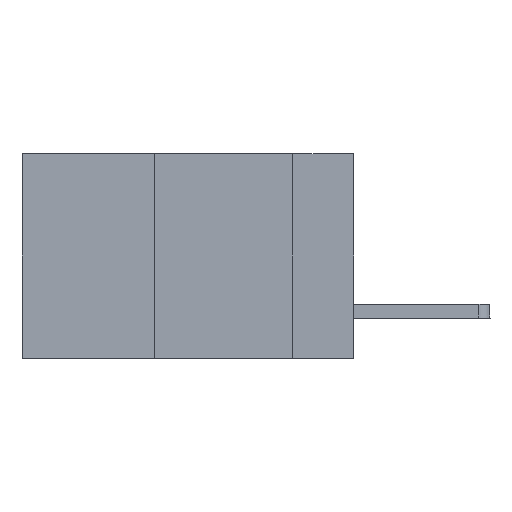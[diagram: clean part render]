
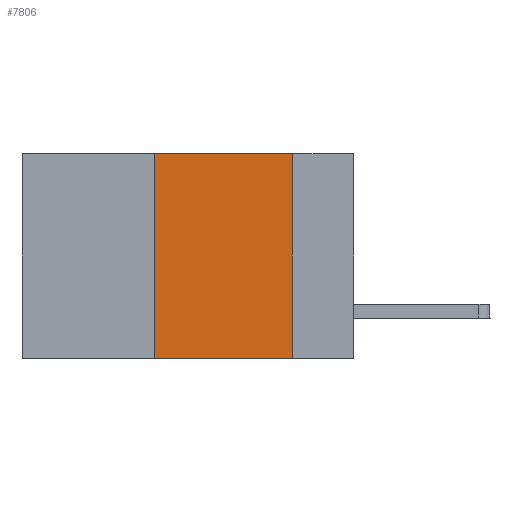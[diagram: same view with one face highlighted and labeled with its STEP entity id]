
A CAD part, left-side view. The second image highlights one B-rep face of the part: STEP entity #7806.
In plain terms, the highlighted planar face has unit normal (-1, 0, 0).
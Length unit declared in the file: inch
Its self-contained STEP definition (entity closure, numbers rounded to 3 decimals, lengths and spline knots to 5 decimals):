
#209 = CARTESIAN_POINT ( 'NONE',  ( 0., 0.11, 0. ) ) ;
#317 = CARTESIAN_POINT ( 'NONE',  ( 0., 0.6, -0.37 ) ) ;
#712 = VECTOR ( 'NONE', #8814, 39.37008 ) ;
#932 = FACE_OUTER_BOUND ( 'NONE', #9823, .T. ) ;
#1489 = LINE ( 'NONE', #3153, #5176 ) ;
#2390 = DIRECTION ( 'NONE',  ( 0., -1., 0. ) ) ;
#2405 = ORIENTED_EDGE ( 'NONE', *, *, #6902, .T. ) ;
#2842 = VERTEX_POINT ( 'NONE', #6450 ) ;
#3153 = CARTESIAN_POINT ( 'NONE',  ( 0., 0.36, 0. ) ) ;
#3265 = CARTESIAN_POINT ( 'NONE',  ( 0., 0.6, 0. ) ) ;
#3742 = VERTEX_POINT ( 'NONE', #10621 ) ;
#4074 = EDGE_CURVE ( 'NONE', #9506, #3742, #1489, .T. ) ;
#4343 = DIRECTION ( 'NONE',  ( 0., 0., -1. ) ) ;
#5105 = LINE ( 'NONE', #317, #13235 ) ;
#5176 = VECTOR ( 'NONE', #10474, 39.37008 ) ;
#5331 = ORIENTED_EDGE ( 'NONE', *, *, #4074, .F. ) ;
#6088 = CARTESIAN_POINT ( 'NONE',  ( 0., 0.6, 0. ) ) ;
#6450 = CARTESIAN_POINT ( 'NONE',  ( 0., 0.11, -0.37 ) ) ;
#6456 = DIRECTION ( 'NONE',  ( 1., 0., 0. ) ) ;
#6552 = VECTOR ( 'NONE', #11394, 39.37008 ) ;
#6637 = ORIENTED_EDGE ( 'NONE', *, *, #10963, .F. ) ;
#6902 = EDGE_CURVE ( 'NONE', #9506, #2842, #5105, .T. ) ;
#7459 = PLANE ( 'NONE',  #12995 ) ;
#7490 = LINE ( 'NONE', #7748, #712 ) ;
#7748 = CARTESIAN_POINT ( 'NONE',  ( 0., 0.11, 0. ) ) ;
#7806 = ADVANCED_FACE ( 'NONE', ( #932 ), #7459, .F. ) ;
#8814 = DIRECTION ( 'NONE',  ( 0., 0., -1. ) ) ;
#9333 = LINE ( 'NONE', #6088, #6552 ) ;
#9506 = VERTEX_POINT ( 'NONE', #12657 ) ;
#9765 = EDGE_CURVE ( 'NONE', #3742, #11503, #9333, .T. ) ;
#9823 = EDGE_LOOP ( 'NONE', ( #6637, #9966, #5331, #2405 ) ) ;
#9966 = ORIENTED_EDGE ( 'NONE', *, *, #9765, .F. ) ;
#10474 = DIRECTION ( 'NONE',  ( 0., 0., 1. ) ) ;
#10621 = CARTESIAN_POINT ( 'NONE',  ( 0., 0.36, 0. ) ) ;
#10963 = EDGE_CURVE ( 'NONE', #11503, #2842, #7490, .T. ) ;
#11394 = DIRECTION ( 'NONE',  ( 0., -1., 0. ) ) ;
#11503 = VERTEX_POINT ( 'NONE', #209 ) ;
#12657 = CARTESIAN_POINT ( 'NONE',  ( 0., 0.36, -0.37 ) ) ;
#12995 = AXIS2_PLACEMENT_3D ( 'NONE', #3265, #6456, #4343 ) ;
#13235 = VECTOR ( 'NONE', #2390, 39.37008 ) ;
